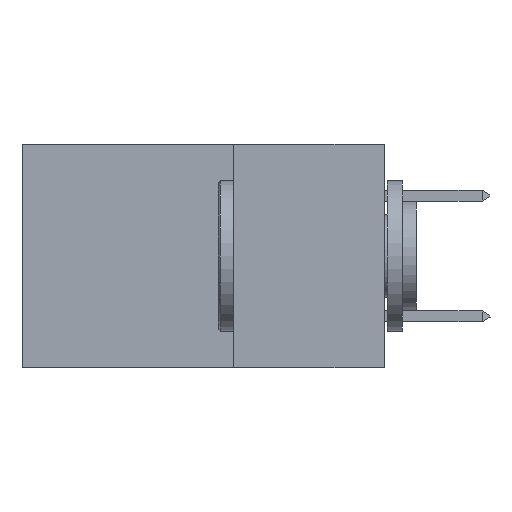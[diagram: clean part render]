
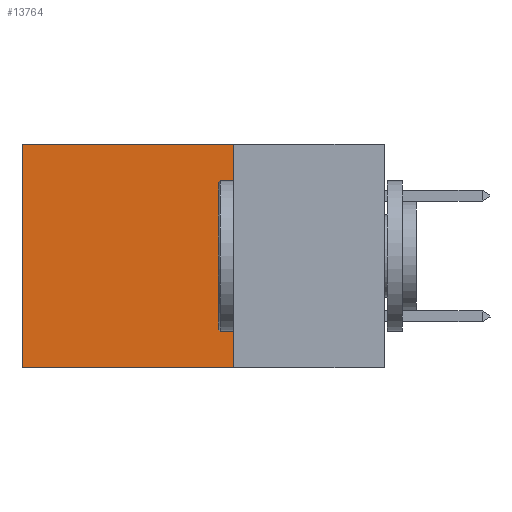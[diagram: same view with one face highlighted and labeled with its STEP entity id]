
A CAD part, left-side view. The second image highlights one B-rep face of the part: STEP entity #13764.
In plain terms, the highlighted planar face has unit normal (-1, 0, 0).
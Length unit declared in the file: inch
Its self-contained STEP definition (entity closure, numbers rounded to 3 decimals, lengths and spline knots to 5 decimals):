
#282 = LINE ( 'NONE', #1621, #25656 ) ;
#599 = DIRECTION ( 'NONE',  ( 0., 0., -1. ) ) ;
#1298 = DIRECTION ( 'NONE',  ( 1., 0., 0. ) ) ;
#1621 = CARTESIAN_POINT ( 'NONE',  ( 0.2875, 0.6, 0. ) ) ;
#2215 = EDGE_CURVE ( 'NONE', #7338, #3737, #17826, .T. ) ;
#2578 = CARTESIAN_POINT ( 'NONE',  ( 0.2875, 0.25, 0. ) ) ;
#2698 = VECTOR ( 'NONE', #16974, 39.37008 ) ;
#3281 = ORIENTED_EDGE ( 'NONE', *, *, #2215, .T. ) ;
#3737 = VERTEX_POINT ( 'NONE', #14050 ) ;
#3996 = CARTESIAN_POINT ( 'NONE',  ( 0.2875, 0.25, 0. ) ) ;
#4353 = LINE ( 'NONE', #2578, #20756 ) ;
#5503 = CARTESIAN_POINT ( 'NONE',  ( 0.2875, 0.25, 0. ) ) ;
#5533 = EDGE_CURVE ( 'NONE', #3737, #13797, #282, .T. ) ;
#7338 = VERTEX_POINT ( 'NONE', #16884 ) ;
#7376 = DIRECTION ( 'NONE',  ( 0., 0., -1. ) ) ;
#12425 = LINE ( 'NONE', #14009, #21106 ) ;
#13764 = ADVANCED_FACE ( 'NONE', ( #22099 ), #17841, .F. ) ;
#13797 = VERTEX_POINT ( 'NONE', #25902 ) ;
#14009 = CARTESIAN_POINT ( 'NONE',  ( 0.2875, 0.25, -0.37 ) ) ;
#14048 = ORIENTED_EDGE ( 'NONE', *, *, #5533, .T. ) ;
#14050 = CARTESIAN_POINT ( 'NONE',  ( 0.2875, 0.6, 0. ) ) ;
#15752 = EDGE_CURVE ( 'NONE', #7338, #21206, #4353, .T. ) ;
#16884 = CARTESIAN_POINT ( 'NONE',  ( 0.2875, 0.25, 0. ) ) ;
#16974 = DIRECTION ( 'NONE',  ( 0., 1., 0. ) ) ;
#17820 = EDGE_LOOP ( 'NONE', ( #14048, #20936, #24192, #3281 ) ) ;
#17826 = LINE ( 'NONE', #3996, #2698 ) ;
#17841 = PLANE ( 'NONE',  #22808 ) ;
#19027 = DIRECTION ( 'NONE',  ( 0., 0., -1. ) ) ;
#20756 = VECTOR ( 'NONE', #19027, 39.37008 ) ;
#20936 = ORIENTED_EDGE ( 'NONE', *, *, #23105, .F. ) ;
#21106 = VECTOR ( 'NONE', #22238, 39.37008 ) ;
#21206 = VERTEX_POINT ( 'NONE', #26400 ) ;
#22099 = FACE_OUTER_BOUND ( 'NONE', #17820, .T. ) ;
#22238 = DIRECTION ( 'NONE',  ( 0., 1., 0. ) ) ;
#22808 = AXIS2_PLACEMENT_3D ( 'NONE', #5503, #1298, #7376 ) ;
#23105 = EDGE_CURVE ( 'NONE', #21206, #13797, #12425, .T. ) ;
#24192 = ORIENTED_EDGE ( 'NONE', *, *, #15752, .F. ) ;
#25656 = VECTOR ( 'NONE', #599, 39.37008 ) ;
#25902 = CARTESIAN_POINT ( 'NONE',  ( 0.2875, 0.6, -0.37 ) ) ;
#26400 = CARTESIAN_POINT ( 'NONE',  ( 0.2875, 0.25, -0.37 ) ) ;
